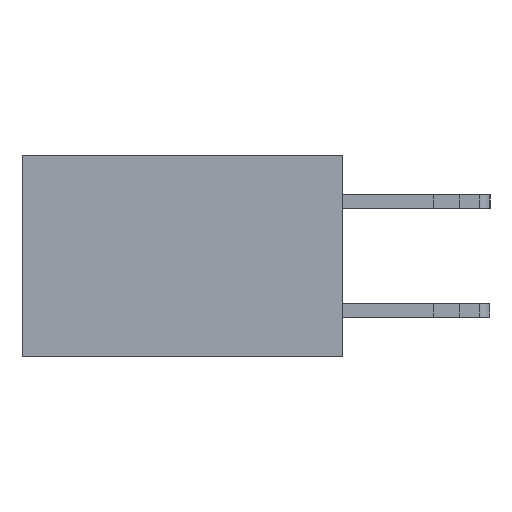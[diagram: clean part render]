
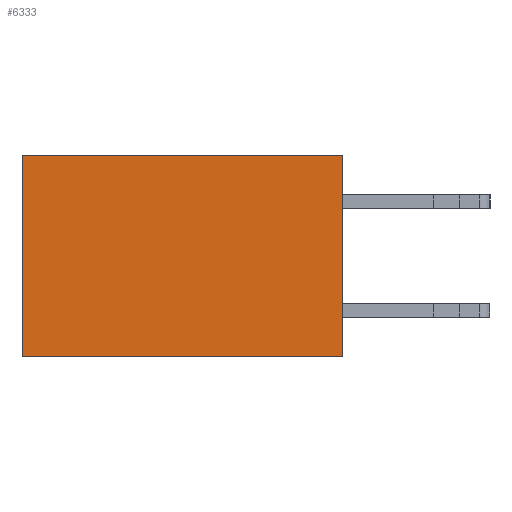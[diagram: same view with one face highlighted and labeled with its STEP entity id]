
A CAD part, left-side view. The second image highlights one B-rep face of the part: STEP entity #6333.
In plain terms, the highlighted planar face has unit normal (-1, 0, 0).
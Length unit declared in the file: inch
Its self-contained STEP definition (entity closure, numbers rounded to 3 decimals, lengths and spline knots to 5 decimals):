
#167 = ORIENTED_EDGE ( 'NONE', *, *, #19892, .F. ) ;
#983 = DIRECTION ( 'NONE',  ( 0., 1., 0. ) ) ;
#2870 = AXIS2_PLACEMENT_3D ( 'NONE', #23348, #23283, #23243 ) ;
#2881 = LINE ( 'NONE', #28345, #9821 ) ;
#5764 = DIRECTION ( 'NONE',  ( 0., 0., -1. ) ) ;
#6254 = FACE_OUTER_BOUND ( 'NONE', #25182, .T. ) ;
#6333 = ADVANCED_FACE ( 'NONE', ( #6254 ), #23456, .F. ) ;
#7592 = LINE ( 'NONE', #20954, #25436 ) ;
#9821 = VECTOR ( 'NONE', #14465, 39.37008 ) ;
#10155 = CARTESIAN_POINT ( 'NONE',  ( 0.277, 0.59, -0.37 ) ) ;
#10262 = CARTESIAN_POINT ( 'NONE',  ( 0.277, 0.59, 0. ) ) ;
#11492 = EDGE_CURVE ( 'NONE', #16921, #12725, #2881, .T. ) ;
#12038 = LINE ( 'NONE', #26732, #24447 ) ;
#12472 = EDGE_CURVE ( 'NONE', #12725, #24367, #7592, .T. ) ;
#12725 = VERTEX_POINT ( 'NONE', #10262 ) ;
#14465 = DIRECTION ( 'NONE',  ( 0., 1., 0. ) ) ;
#14700 = ORIENTED_EDGE ( 'NONE', *, *, #17224, .F. ) ;
#15077 = CARTESIAN_POINT ( 'NONE',  ( 0.277, 0., -0.37 ) ) ;
#16921 = VERTEX_POINT ( 'NONE', #27854 ) ;
#17224 = EDGE_CURVE ( 'NONE', #18169, #24367, #24925, .T. ) ;
#18054 = CARTESIAN_POINT ( 'NONE',  ( 0.277, 0., -0.37 ) ) ;
#18169 = VERTEX_POINT ( 'NONE', #18054 ) ;
#18607 = DIRECTION ( 'NONE',  ( 0., 0., -1. ) ) ;
#19311 = ORIENTED_EDGE ( 'NONE', *, *, #11492, .T. ) ;
#19892 = EDGE_CURVE ( 'NONE', #16921, #18169, #12038, .T. ) ;
#20954 = CARTESIAN_POINT ( 'NONE',  ( 0.277, 0.59, -0.37 ) ) ;
#23243 = DIRECTION ( 'NONE',  ( 0., 0., -1. ) ) ;
#23283 = DIRECTION ( 'NONE',  ( 1., 0., 0. ) ) ;
#23348 = CARTESIAN_POINT ( 'NONE',  ( 0.277, 0., -0.37 ) ) ;
#23456 = PLANE ( 'NONE',  #2870 ) ;
#24367 = VERTEX_POINT ( 'NONE', #10155 ) ;
#24447 = VECTOR ( 'NONE', #5764, 39.37008 ) ;
#24866 = ORIENTED_EDGE ( 'NONE', *, *, #12472, .T. ) ;
#24925 = LINE ( 'NONE', #15077, #25628 ) ;
#25182 = EDGE_LOOP ( 'NONE', ( #24866, #14700, #167, #19311 ) ) ;
#25436 = VECTOR ( 'NONE', #18607, 39.37008 ) ;
#25628 = VECTOR ( 'NONE', #983, 39.37008 ) ;
#26732 = CARTESIAN_POINT ( 'NONE',  ( 0.277, 0., -0.37 ) ) ;
#27854 = CARTESIAN_POINT ( 'NONE',  ( 0.277, 0., 0. ) ) ;
#28345 = CARTESIAN_POINT ( 'NONE',  ( 0.277, 0., 0. ) ) ;
